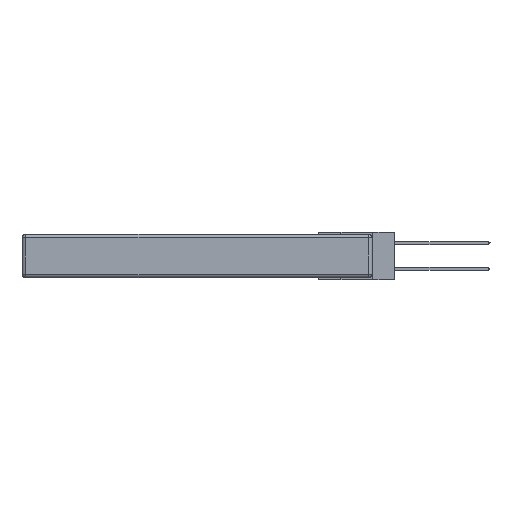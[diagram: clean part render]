
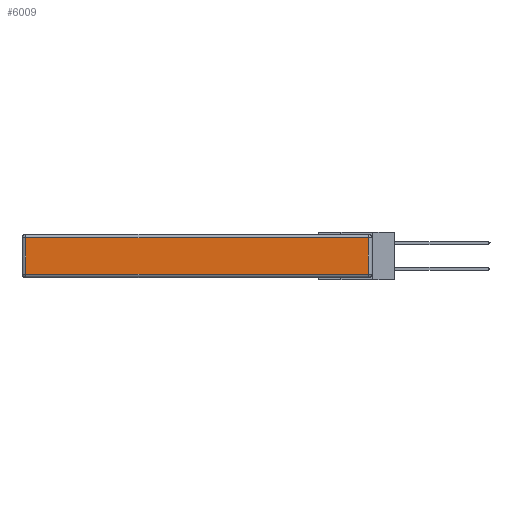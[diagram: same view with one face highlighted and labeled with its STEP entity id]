
A CAD part, left-side view. The second image highlights one B-rep face of the part: STEP entity #6009.
In plain terms, the highlighted planar face has unit normal (-1, 0, 0).
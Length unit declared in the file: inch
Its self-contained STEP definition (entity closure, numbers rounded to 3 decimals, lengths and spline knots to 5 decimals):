
#375 = LINE ( 'NONE', #16956, #8295 ) ;
#728 = EDGE_CURVE ( 'NONE', #21796, #15871, #375, .T. ) ;
#1190 = CARTESIAN_POINT ( 'NONE',  ( 0., 2.72, -0.313 ) ) ;
#1325 = VERTEX_POINT ( 'NONE', #25744 ) ;
#3088 = PLANE ( 'NONE',  #17497 ) ;
#3154 = DIRECTION ( 'NONE',  ( 0., 0., -1. ) ) ;
#3604 = ORIENTED_EDGE ( 'NONE', *, *, #728, .T. ) ;
#5176 = CARTESIAN_POINT ( 'NONE',  ( 0., 2.72, -0.343 ) ) ;
#6009 = ADVANCED_FACE ( 'NONE', ( #23647 ), #3088, .T. ) ;
#7522 = CARTESIAN_POINT ( 'NONE',  ( 0., 0., -0.343 ) ) ;
#8295 = VECTOR ( 'NONE', #24899, 39.37008 ) ;
#9111 = VECTOR ( 'NONE', #22254, 39.37008 ) ;
#11261 = CARTESIAN_POINT ( 'NONE',  ( 0., 0., -0.313 ) ) ;
#11482 = DIRECTION ( 'NONE',  ( -1., 0., 0. ) ) ;
#11824 = EDGE_CURVE ( 'NONE', #1325, #21796, #20482, .T. ) ;
#12740 = EDGE_LOOP ( 'NONE', ( #20483, #23749, #3604, #22666 ) ) ;
#14971 = VECTOR ( 'NONE', #3154, 39.37008 ) ;
#15058 = EDGE_CURVE ( 'NONE', #15871, #19210, #20471, .T. ) ;
#15663 = VECTOR ( 'NONE', #23378, 39.37008 ) ;
#15871 = VERTEX_POINT ( 'NONE', #18598 ) ;
#16956 = CARTESIAN_POINT ( 'NONE',  ( 0., 2.75, -0.03 ) ) ;
#16976 = LINE ( 'NONE', #11261, #15663 ) ;
#17497 = AXIS2_PLACEMENT_3D ( 'NONE', #7522, #11482, #26283 ) ;
#18176 = CARTESIAN_POINT ( 'NONE',  ( 0., 0.03, -0.343 ) ) ;
#18598 = CARTESIAN_POINT ( 'NONE',  ( 0., 2.72, -0.03 ) ) ;
#19210 = VERTEX_POINT ( 'NONE', #1190 ) ;
#19988 = CARTESIAN_POINT ( 'NONE',  ( 0., 0.03, -0.03 ) ) ;
#20133 = EDGE_CURVE ( 'NONE', #19210, #1325, #16976, .T. ) ;
#20471 = LINE ( 'NONE', #5176, #14971 ) ;
#20482 = LINE ( 'NONE', #18176, #9111 ) ;
#20483 = ORIENTED_EDGE ( 'NONE', *, *, #20133, .T. ) ;
#21796 = VERTEX_POINT ( 'NONE', #19988 ) ;
#22254 = DIRECTION ( 'NONE',  ( 0., 0., 1. ) ) ;
#22666 = ORIENTED_EDGE ( 'NONE', *, *, #15058, .T. ) ;
#23378 = DIRECTION ( 'NONE',  ( 0., -1., 0. ) ) ;
#23647 = FACE_OUTER_BOUND ( 'NONE', #12740, .T. ) ;
#23749 = ORIENTED_EDGE ( 'NONE', *, *, #11824, .T. ) ;
#24899 = DIRECTION ( 'NONE',  ( 0., 1., 0. ) ) ;
#25744 = CARTESIAN_POINT ( 'NONE',  ( 0., 0.03, -0.313 ) ) ;
#26283 = DIRECTION ( 'NONE',  ( 0., 0., 1. ) ) ;
